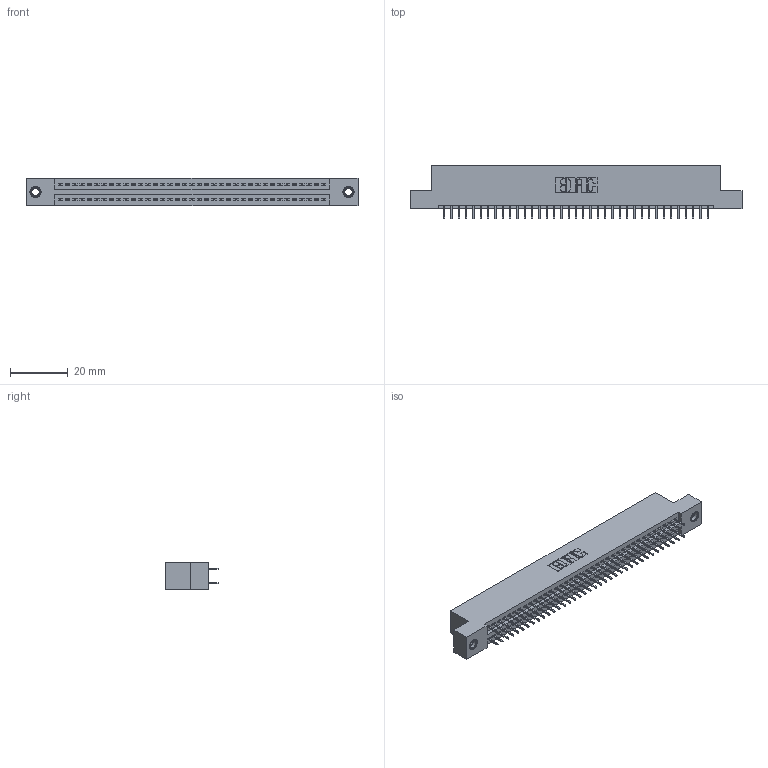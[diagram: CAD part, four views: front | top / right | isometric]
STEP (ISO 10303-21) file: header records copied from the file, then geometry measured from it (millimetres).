
FILE_DESCRIPTION (( 'STEP AP203' ), '1' );
FILE_NAME ('395-074-525-207.STEP', '2020-09-25T08:23:07', ( '' ), ( '' ), 'SwSTEP 2.0', 'SolidWorks 2020', '' );
FILE_SCHEMA (( 'CONFIG_CONTROL_DESIGN' ));
Length unit declared in the file: inch
Products named in the file (4): 395-074-525-207; 345-250-001_345-250-005-103; 345 Part_Flush Mounting Lugs - 0.156 Dia-TI; 345-292-001_345-293-125
Assembly tree (77 placements, depth 2):
  395-074-525-207
    345 Part_Flush Mounting Lugs - 0.156 Dia-TI
    345-292-001_345-293-125  x74
    345-250-001_345-250-005-103  x2
Bounding box: 115.19 x 18.72 x 9.4 mm (x, y, z)
Volume: 11007.8 mm3; surface area: 15835.4 mm2
Topology: 77 solids, 77 shells, 4182 faces, 11799 edges, 7562 vertices
Faces by surface type: plane 2998, cylinder 1168, cone 12, torus 4
Entity records: 30964 total; most frequent: CARTESIAN_POINT 5175, ORIENTED_EDGE 5102, DIRECTION 4597, EDGE_CURVE 2551, VECTOR 2255, LINE 2255, VERTEX_POINT 1692, AXIS2_PLACEMENT_3D 1171
